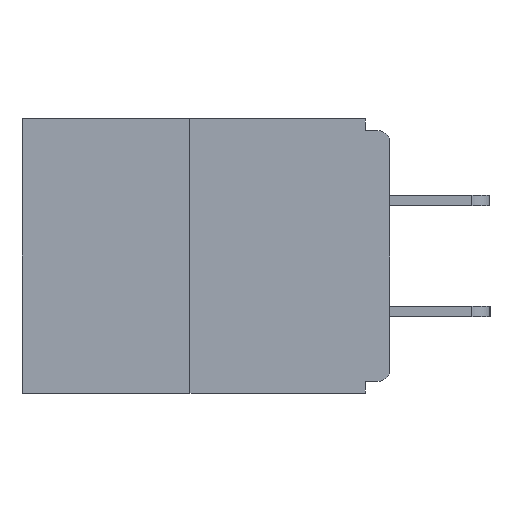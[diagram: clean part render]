
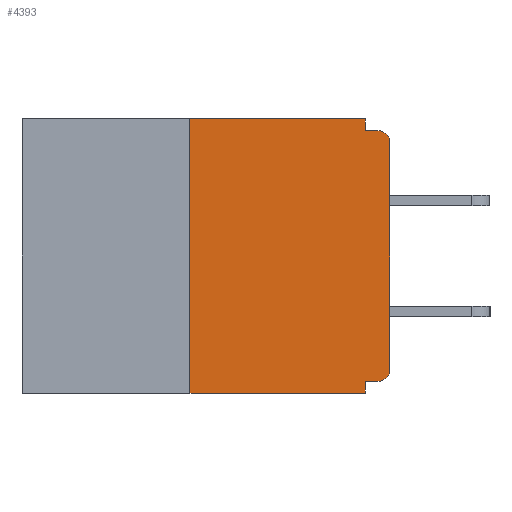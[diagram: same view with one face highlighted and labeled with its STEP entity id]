
A CAD part, left-side view. The second image highlights one B-rep face of the part: STEP entity #4393.
In plain terms, the highlighted planar face has unit normal (-1, 0, 0).
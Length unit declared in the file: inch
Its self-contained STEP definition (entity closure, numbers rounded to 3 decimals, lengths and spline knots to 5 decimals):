
#170 = LINE ( 'NONE', #13682, #6926 ) ;
#237 = VERTEX_POINT ( 'NONE', #2183 ) ;
#496 = EDGE_CURVE ( 'NONE', #17672, #237, #1708, .T. ) ;
#642 = CARTESIAN_POINT ( 'NONE',  ( 0., 0., -0.015 ) ) ;
#672 = VERTEX_POINT ( 'NONE', #9048 ) ;
#1038 = DIRECTION ( 'NONE',  ( 0., 0., -1. ) ) ;
#1540 = ORIENTED_EDGE ( 'NONE', *, *, #13654, .T. ) ;
#1571 = EDGE_CURVE ( 'NONE', #13820, #2654, #17612, .T. ) ;
#1609 = LINE ( 'NONE', #642, #10708 ) ;
#1708 = LINE ( 'NONE', #3239, #4953 ) ;
#1776 = DIRECTION ( 'NONE',  ( 0., 0., 1. ) ) ;
#1970 = VERTEX_POINT ( 'NONE', #15161 ) ;
#2130 = VERTEX_POINT ( 'NONE', #2777 ) ;
#2155 = DIRECTION ( 'NONE',  ( -1., 0., 0. ) ) ;
#2183 = CARTESIAN_POINT ( 'NONE',  ( 0., 0.031, -0.015 ) ) ;
#2285 = CIRCLE ( 'NONE', #6335, 0.015 ) ;
#2494 = CARTESIAN_POINT ( 'NONE',  ( 0., 0., -0.328 ) ) ;
#2647 = EDGE_CURVE ( 'NONE', #4520, #672, #10759, .T. ) ;
#2654 = VERTEX_POINT ( 'NONE', #16631 ) ;
#2777 = CARTESIAN_POINT ( 'NONE',  ( 0., 0.031, -0.328 ) ) ;
#2780 = AXIS2_PLACEMENT_3D ( 'NONE', #15687, #2155, #16194 ) ;
#2886 = VECTOR ( 'NONE', #9305, 39.37008 ) ;
#2957 = VERTEX_POINT ( 'NONE', #12199 ) ;
#3239 = CARTESIAN_POINT ( 'NONE',  ( 0., 0.031, 0. ) ) ;
#3756 = DIRECTION ( 'NONE',  ( 1., 0., 0. ) ) ;
#3886 = EDGE_CURVE ( 'NONE', #1970, #13820, #6542, .T. ) ;
#4393 = ADVANCED_FACE ( 'NONE', ( #17722 ), #12465, .F. ) ;
#4520 = VERTEX_POINT ( 'NONE', #16885 ) ;
#4871 = ORIENTED_EDGE ( 'NONE', *, *, #3886, .T. ) ;
#4953 = VECTOR ( 'NONE', #15666, 39.37008 ) ;
#5323 = AXIS2_PLACEMENT_3D ( 'NONE', #16344, #3756, #1038 ) ;
#5389 = ORIENTED_EDGE ( 'NONE', *, *, #17321, .F. ) ;
#6335 = AXIS2_PLACEMENT_3D ( 'NONE', #8641, #12819, #17257 ) ;
#6542 = CIRCLE ( 'NONE', #2780, 0.015 ) ;
#6926 = VECTOR ( 'NONE', #13759, 39.37008 ) ;
#7357 = ORIENTED_EDGE ( 'NONE', *, *, #9145, .F. ) ;
#7871 = CARTESIAN_POINT ( 'NONE',  ( 0., 0.46, 0. ) ) ;
#7874 = VECTOR ( 'NONE', #11111, 39.37008 ) ;
#8033 = LINE ( 'NONE', #2494, #15007 ) ;
#8324 = EDGE_CURVE ( 'NONE', #1970, #2130, #8033, .T. ) ;
#8641 = CARTESIAN_POINT ( 'NONE',  ( 0., 0.015, -0.03 ) ) ;
#8890 = CARTESIAN_POINT ( 'NONE',  ( 0., 0.25, 0. ) ) ;
#9048 = CARTESIAN_POINT ( 'NONE',  ( 0., 0.031, -0.343 ) ) ;
#9145 = EDGE_CURVE ( 'NONE', #2130, #672, #170, .T. ) ;
#9305 = DIRECTION ( 'NONE',  ( 0., -1., 0. ) ) ;
#9307 = DIRECTION ( 'NONE',  ( 0., 1., 0. ) ) ;
#9334 = EDGE_CURVE ( 'NONE', #237, #2957, #1609, .T. ) ;
#10293 = VECTOR ( 'NONE', #17708, 39.37008 ) ;
#10708 = VECTOR ( 'NONE', #11416, 39.37008 ) ;
#10759 = LINE ( 'NONE', #13828, #7874 ) ;
#10883 = VECTOR ( 'NONE', #1776, 39.37008 ) ;
#11111 = DIRECTION ( 'NONE',  ( 0., -1., 0. ) ) ;
#11190 = CARTESIAN_POINT ( 'NONE',  ( 0., 0.25, 0. ) ) ;
#11416 = DIRECTION ( 'NONE',  ( 0., -1., 0. ) ) ;
#11472 = LINE ( 'NONE', #11190, #10883 ) ;
#11706 = VERTEX_POINT ( 'NONE', #8890 ) ;
#12199 = CARTESIAN_POINT ( 'NONE',  ( 0., 0.015, -0.015 ) ) ;
#12465 = PLANE ( 'NONE',  #5323 ) ;
#12819 = DIRECTION ( 'NONE',  ( -1., 0., 0. ) ) ;
#13437 = CARTESIAN_POINT ( 'NONE',  ( 0., 0., 0. ) ) ;
#13654 = EDGE_CURVE ( 'NONE', #2654, #2957, #2285, .T. ) ;
#13682 = CARTESIAN_POINT ( 'NONE',  ( 0., 0.031, -0.343 ) ) ;
#13759 = DIRECTION ( 'NONE',  ( 0., 0., -1. ) ) ;
#13820 = VERTEX_POINT ( 'NONE', #16814 ) ;
#13828 = CARTESIAN_POINT ( 'NONE',  ( 0., 0.46, -0.343 ) ) ;
#13916 = ORIENTED_EDGE ( 'NONE', *, *, #1571, .T. ) ;
#14749 = LINE ( 'NONE', #7871, #2886 ) ;
#15007 = VECTOR ( 'NONE', #9307, 39.37008 ) ;
#15161 = CARTESIAN_POINT ( 'NONE',  ( 0., 0.015, -0.328 ) ) ;
#15212 = ORIENTED_EDGE ( 'NONE', *, *, #9334, .F. ) ;
#15444 = ORIENTED_EDGE ( 'NONE', *, *, #17111, .F. ) ;
#15666 = DIRECTION ( 'NONE',  ( 0., 0., -1. ) ) ;
#15687 = CARTESIAN_POINT ( 'NONE',  ( 0., 0.015, -0.313 ) ) ;
#16194 = DIRECTION ( 'NONE',  ( 0., 0., -1. ) ) ;
#16343 = CARTESIAN_POINT ( 'NONE',  ( 0., 0.031, 0. ) ) ;
#16344 = CARTESIAN_POINT ( 'NONE',  ( 0., 0.46, 0. ) ) ;
#16631 = CARTESIAN_POINT ( 'NONE',  ( 0., 0., -0.03 ) ) ;
#16732 = ORIENTED_EDGE ( 'NONE', *, *, #8324, .F. ) ;
#16814 = CARTESIAN_POINT ( 'NONE',  ( 0., 0., -0.313 ) ) ;
#16885 = CARTESIAN_POINT ( 'NONE',  ( 0., 0.25, -0.343 ) ) ;
#16960 = ORIENTED_EDGE ( 'NONE', *, *, #496, .F. ) ;
#17111 = EDGE_CURVE ( 'NONE', #11706, #17672, #14749, .T. ) ;
#17257 = DIRECTION ( 'NONE',  ( 0., 0., -1. ) ) ;
#17321 = EDGE_CURVE ( 'NONE', #4520, #11706, #11472, .T. ) ;
#17415 = EDGE_LOOP ( 'NONE', ( #15444, #5389, #17716, #7357, #16732, #4871, #13916, #1540, #15212, #16960 ) ) ;
#17612 = LINE ( 'NONE', #13437, #10293 ) ;
#17672 = VERTEX_POINT ( 'NONE', #16343 ) ;
#17708 = DIRECTION ( 'NONE',  ( 0., 0., 1. ) ) ;
#17716 = ORIENTED_EDGE ( 'NONE', *, *, #2647, .T. ) ;
#17722 = FACE_OUTER_BOUND ( 'NONE', #17415, .T. ) ;
